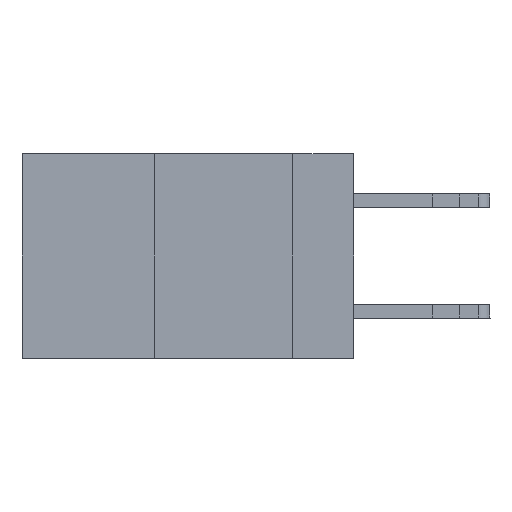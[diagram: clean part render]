
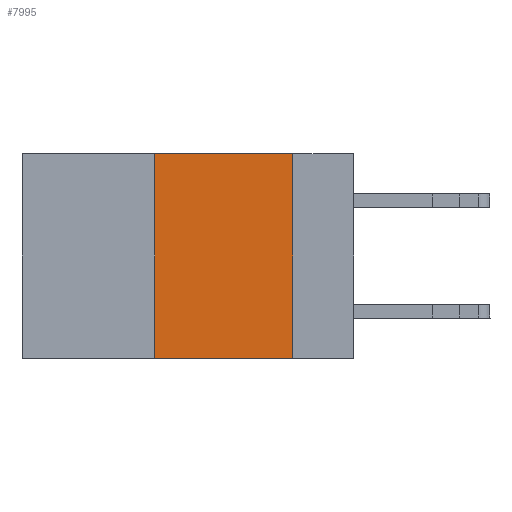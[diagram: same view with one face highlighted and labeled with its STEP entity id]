
A CAD part, left-side view. The second image highlights one B-rep face of the part: STEP entity #7995.
In plain terms, the highlighted planar face has unit normal (-1, 0, 0).
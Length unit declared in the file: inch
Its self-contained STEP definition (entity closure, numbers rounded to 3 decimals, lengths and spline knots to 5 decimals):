
#254 = DIRECTION ( 'NONE',  ( 1., 0., 0. ) ) ;
#527 = EDGE_CURVE ( 'NONE', #11685, #20349, #12249, .T. ) ;
#1385 = ORIENTED_EDGE ( 'NONE', *, *, #527, .F. ) ;
#1409 = DIRECTION ( 'NONE',  ( 0., 0., 1. ) ) ;
#1696 = FACE_OUTER_BOUND ( 'NONE', #5476, .T. ) ;
#1699 = AXIS2_PLACEMENT_3D ( 'NONE', #11326, #254, #17944 ) ;
#2410 = EDGE_CURVE ( 'NONE', #15529, #2575, #9575, .T. ) ;
#2575 = VERTEX_POINT ( 'NONE', #20152 ) ;
#2839 = CARTESIAN_POINT ( 'NONE',  ( 0., 0.11, 0. ) ) ;
#3071 = VECTOR ( 'NONE', #20545, 39.37008 ) ;
#4465 = CARTESIAN_POINT ( 'NONE',  ( 0., 0.11, 0. ) ) ;
#5476 = EDGE_LOOP ( 'NONE', ( #12035, #8481, #1385, #20474 ) ) ;
#7616 = VECTOR ( 'NONE', #1409, 39.37008 ) ;
#7966 = EDGE_CURVE ( 'NONE', #20349, #15529, #16268, .T. ) ;
#7995 = ADVANCED_FACE ( 'NONE', ( #1696 ), #8097, .F. ) ;
#8074 = LINE ( 'NONE', #12978, #3071 ) ;
#8097 = PLANE ( 'NONE',  #1699 ) ;
#8481 = ORIENTED_EDGE ( 'NONE', *, *, #7966, .F. ) ;
#9325 = CARTESIAN_POINT ( 'NONE',  ( 0., 0.36, -0.37 ) ) ;
#9575 = LINE ( 'NONE', #4465, #11905 ) ;
#11326 = CARTESIAN_POINT ( 'NONE',  ( 0., 0.6, 0. ) ) ;
#11685 = VERTEX_POINT ( 'NONE', #9325 ) ;
#11905 = VECTOR ( 'NONE', #12291, 39.37008 ) ;
#12035 = ORIENTED_EDGE ( 'NONE', *, *, #2410, .F. ) ;
#12249 = LINE ( 'NONE', #20477, #7616 ) ;
#12291 = DIRECTION ( 'NONE',  ( 0., 0., -1. ) ) ;
#12978 = CARTESIAN_POINT ( 'NONE',  ( 0., 0.6, -0.37 ) ) ;
#13098 = DIRECTION ( 'NONE',  ( 0., -1., 0. ) ) ;
#13731 = VECTOR ( 'NONE', #13098, 39.37008 ) ;
#13732 = EDGE_CURVE ( 'NONE', #11685, #2575, #8074, .T. ) ;
#15529 = VERTEX_POINT ( 'NONE', #2839 ) ;
#16268 = LINE ( 'NONE', #19625, #13731 ) ;
#17944 = DIRECTION ( 'NONE',  ( 0., 0., -1. ) ) ;
#19625 = CARTESIAN_POINT ( 'NONE',  ( 0., 0.6, 0. ) ) ;
#19921 = CARTESIAN_POINT ( 'NONE',  ( 0., 0.36, 0. ) ) ;
#20152 = CARTESIAN_POINT ( 'NONE',  ( 0., 0.11, -0.37 ) ) ;
#20349 = VERTEX_POINT ( 'NONE', #19921 ) ;
#20474 = ORIENTED_EDGE ( 'NONE', *, *, #13732, .T. ) ;
#20477 = CARTESIAN_POINT ( 'NONE',  ( 0., 0.36, 0. ) ) ;
#20545 = DIRECTION ( 'NONE',  ( 0., -1., 0. ) ) ;
